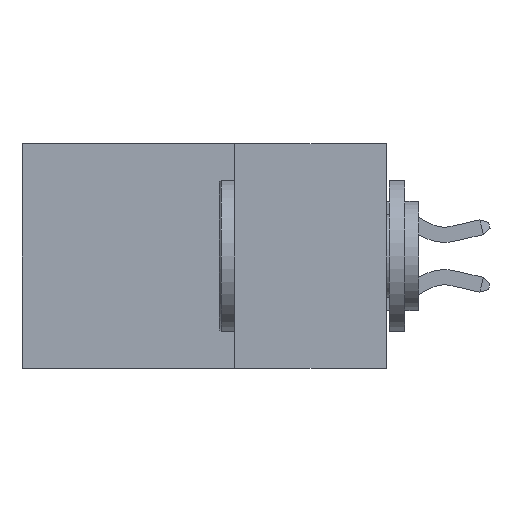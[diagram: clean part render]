
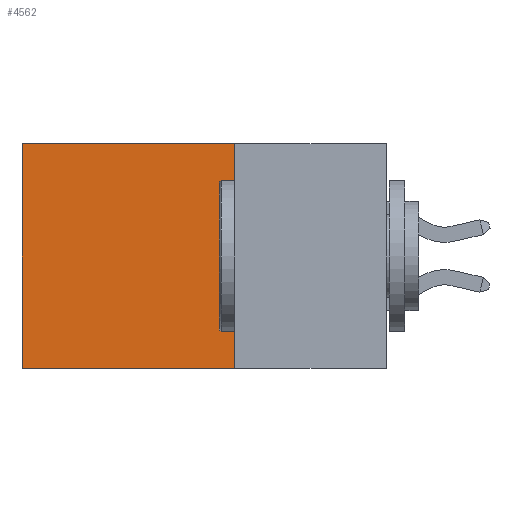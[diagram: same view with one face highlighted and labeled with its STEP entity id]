
A CAD part, left-side view. The second image highlights one B-rep face of the part: STEP entity #4562.
In plain terms, the highlighted planar face has unit normal (-1, 0, 0).
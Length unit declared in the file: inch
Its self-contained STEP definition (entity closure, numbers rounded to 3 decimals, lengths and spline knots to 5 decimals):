
#820 = CARTESIAN_POINT ( 'NONE',  ( 0.2615, 0.25, 0. ) ) ;
#1442 = VERTEX_POINT ( 'NONE', #6061 ) ;
#2519 = CARTESIAN_POINT ( 'NONE',  ( 0.2615, 0.25, -0.37 ) ) ;
#3389 = FACE_OUTER_BOUND ( 'NONE', #20001, .T. ) ;
#3680 = CARTESIAN_POINT ( 'NONE',  ( 0.2615, 0.6, 0. ) ) ;
#3780 = VERTEX_POINT ( 'NONE', #820 ) ;
#4562 = ADVANCED_FACE ( 'NONE', ( #3389 ), #7870, .F. ) ;
#4609 = ORIENTED_EDGE ( 'NONE', *, *, #13365, .T. ) ;
#5593 = VERTEX_POINT ( 'NONE', #3680 ) ;
#5604 = DIRECTION ( 'NONE',  ( 0., 0., -1. ) ) ;
#5753 = VECTOR ( 'NONE', #23455, 39.37008 ) ;
#6061 = CARTESIAN_POINT ( 'NONE',  ( 0.2615, 0.25, -0.37 ) ) ;
#6654 = DIRECTION ( 'NONE',  ( 0., 0., -1. ) ) ;
#7665 = CARTESIAN_POINT ( 'NONE',  ( 0.2615, 0.25, 0. ) ) ;
#7797 = LINE ( 'NONE', #2519, #15066 ) ;
#7870 = PLANE ( 'NONE',  #8014 ) ;
#8014 = AXIS2_PLACEMENT_3D ( 'NONE', #13656, #11592, #23286 ) ;
#9391 = EDGE_CURVE ( 'NONE', #1442, #15350, #7797, .T. ) ;
#11009 = ORIENTED_EDGE ( 'NONE', *, *, #17616, .F. ) ;
#11128 = CARTESIAN_POINT ( 'NONE',  ( 0.2615, 0.6, -0.37 ) ) ;
#11592 = DIRECTION ( 'NONE',  ( 1., 0., 0. ) ) ;
#12174 = CARTESIAN_POINT ( 'NONE',  ( 0.2615, 0.6, -0.37 ) ) ;
#12750 = VECTOR ( 'NONE', #5604, 39.37008 ) ;
#13365 = EDGE_CURVE ( 'NONE', #5593, #15350, #22818, .T. ) ;
#13411 = VECTOR ( 'NONE', #6654, 39.37008 ) ;
#13656 = CARTESIAN_POINT ( 'NONE',  ( 0.2615, 0.25, -0.37 ) ) ;
#13952 = DIRECTION ( 'NONE',  ( 0., 1., 0. ) ) ;
#15066 = VECTOR ( 'NONE', #13952, 39.37008 ) ;
#15350 = VERTEX_POINT ( 'NONE', #12174 ) ;
#15739 = LINE ( 'NONE', #7665, #5753 ) ;
#16782 = ORIENTED_EDGE ( 'NONE', *, *, #18999, .T. ) ;
#17616 = EDGE_CURVE ( 'NONE', #3780, #1442, #23188, .T. ) ;
#18999 = EDGE_CURVE ( 'NONE', #3780, #5593, #15739, .T. ) ;
#20001 = EDGE_LOOP ( 'NONE', ( #4609, #20519, #11009, #16782 ) ) ;
#20519 = ORIENTED_EDGE ( 'NONE', *, *, #9391, .F. ) ;
#21514 = CARTESIAN_POINT ( 'NONE',  ( 0.2615, 0.25, -0.37 ) ) ;
#22818 = LINE ( 'NONE', #11128, #13411 ) ;
#23188 = LINE ( 'NONE', #21514, #12750 ) ;
#23286 = DIRECTION ( 'NONE',  ( 0., 0., -1. ) ) ;
#23455 = DIRECTION ( 'NONE',  ( 0., 1., 0. ) ) ;
